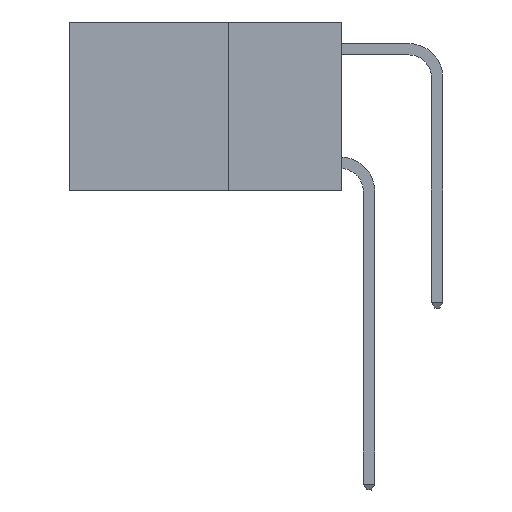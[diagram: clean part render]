
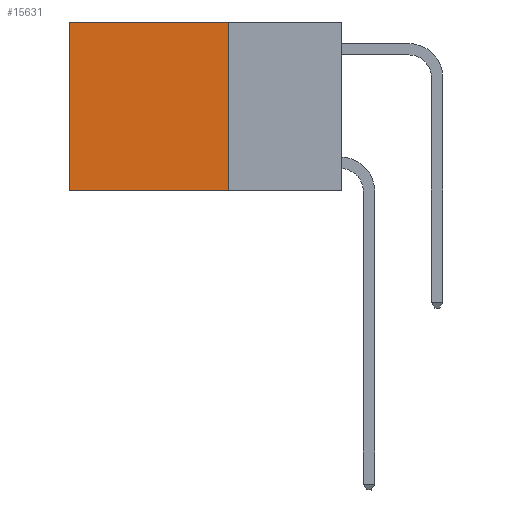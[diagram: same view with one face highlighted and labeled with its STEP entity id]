
A CAD part, left-side view. The second image highlights one B-rep face of the part: STEP entity #15631.
In plain terms, the highlighted planar face has unit normal (-1, 0, 0).
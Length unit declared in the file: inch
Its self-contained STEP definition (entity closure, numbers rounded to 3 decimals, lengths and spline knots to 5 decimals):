
#361 = LINE ( 'NONE', #7323, #30727 ) ;
#515 = VECTOR ( 'NONE', #28039, 39.37008 ) ;
#540 = ORIENTED_EDGE ( 'NONE', *, *, #28943, .F. ) ;
#1896 = VERTEX_POINT ( 'NONE', #28600 ) ;
#2152 = ORIENTED_EDGE ( 'NONE', *, *, #25600, .F. ) ;
#2258 = EDGE_LOOP ( 'NONE', ( #18222, #540, #2152, #3824 ) ) ;
#2392 = VERTEX_POINT ( 'NONE', #23822 ) ;
#3533 = CARTESIAN_POINT ( 'NONE',  ( 0.2625, 0.6, 0. ) ) ;
#3824 = ORIENTED_EDGE ( 'NONE', *, *, #5768, .T. ) ;
#4863 = PLANE ( 'NONE',  #6184 ) ;
#5768 = EDGE_CURVE ( 'NONE', #14147, #21254, #23293, .T. ) ;
#6184 = AXIS2_PLACEMENT_3D ( 'NONE', #11957, #29182, #7525 ) ;
#7323 = CARTESIAN_POINT ( 'NONE',  ( 0.2625, 0.25, -0.37 ) ) ;
#7525 = DIRECTION ( 'NONE',  ( 0., 0., -1. ) ) ;
#9691 = DIRECTION ( 'NONE',  ( 0., 1., 0. ) ) ;
#9896 = FACE_OUTER_BOUND ( 'NONE', #2258, .T. ) ;
#11957 = CARTESIAN_POINT ( 'NONE',  ( 0.2625, 0.25, 0. ) ) ;
#12707 = CARTESIAN_POINT ( 'NONE',  ( 0.2625, 0.25, 0. ) ) ;
#13015 = LINE ( 'NONE', #12707, #14624 ) ;
#14147 = VERTEX_POINT ( 'NONE', #22927 ) ;
#14235 = EDGE_CURVE ( 'NONE', #21254, #1896, #25167, .T. ) ;
#14624 = VECTOR ( 'NONE', #19646, 39.37008 ) ;
#15062 = DIRECTION ( 'NONE',  ( 0., 0., -1. ) ) ;
#15631 = ADVANCED_FACE ( 'NONE', ( #9896 ), #4863, .F. ) ;
#18222 = ORIENTED_EDGE ( 'NONE', *, *, #14235, .T. ) ;
#18409 = CARTESIAN_POINT ( 'NONE',  ( 0.2625, 0.25, 0. ) ) ;
#19646 = DIRECTION ( 'NONE',  ( 0., 0., -1. ) ) ;
#21254 = VERTEX_POINT ( 'NONE', #24071 ) ;
#22927 = CARTESIAN_POINT ( 'NONE',  ( 0.2625, 0.25, 0. ) ) ;
#23293 = LINE ( 'NONE', #18409, #515 ) ;
#23822 = CARTESIAN_POINT ( 'NONE',  ( 0.2625, 0.25, -0.37 ) ) ;
#24071 = CARTESIAN_POINT ( 'NONE',  ( 0.2625, 0.6, 0. ) ) ;
#24367 = VECTOR ( 'NONE', #15062, 39.37008 ) ;
#25167 = LINE ( 'NONE', #3533, #24367 ) ;
#25600 = EDGE_CURVE ( 'NONE', #14147, #2392, #13015, .T. ) ;
#28039 = DIRECTION ( 'NONE',  ( 0., 1., 0. ) ) ;
#28600 = CARTESIAN_POINT ( 'NONE',  ( 0.2625, 0.6, -0.37 ) ) ;
#28943 = EDGE_CURVE ( 'NONE', #2392, #1896, #361, .T. ) ;
#29182 = DIRECTION ( 'NONE',  ( 1., 0., 0. ) ) ;
#30727 = VECTOR ( 'NONE', #9691, 39.37008 ) ;
